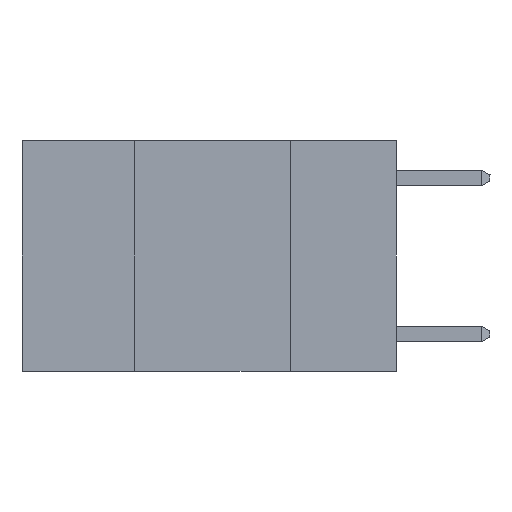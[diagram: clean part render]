
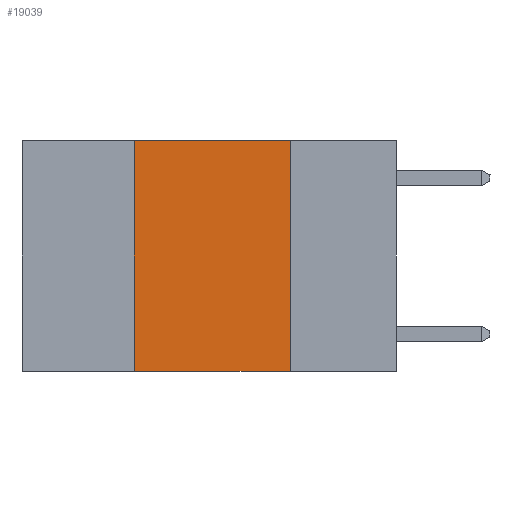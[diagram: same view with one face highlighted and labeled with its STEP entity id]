
A CAD part, left-side view. The second image highlights one B-rep face of the part: STEP entity #19039.
In plain terms, the highlighted planar face has unit normal (-1, 0, 0).
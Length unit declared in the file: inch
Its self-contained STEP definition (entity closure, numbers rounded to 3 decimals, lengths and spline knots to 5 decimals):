
#1500 = CARTESIAN_POINT ( 'NONE',  ( 0., 0.6, -0.37 ) ) ;
#1805 = EDGE_CURVE ( 'NONE', #14149, #16679, #2577, .T. ) ;
#2020 = CARTESIAN_POINT ( 'NONE',  ( 0., 0.42, -0.37 ) ) ;
#2577 = LINE ( 'NONE', #16884, #18475 ) ;
#2662 = ORIENTED_EDGE ( 'NONE', *, *, #11270, .T. ) ;
#3321 = LINE ( 'NONE', #1500, #19253 ) ;
#4371 = CARTESIAN_POINT ( 'NONE',  ( 0., 0.42, 0. ) ) ;
#4613 = DIRECTION ( 'NONE',  ( 0., -1., 0. ) ) ;
#5341 = VECTOR ( 'NONE', #7703, 39.37008 ) ;
#5435 = EDGE_CURVE ( 'NONE', #5509, #14876, #9414, .T. ) ;
#5509 = VERTEX_POINT ( 'NONE', #14030 ) ;
#7008 = EDGE_CURVE ( 'NONE', #16679, #5509, #19397, .T. ) ;
#7703 = DIRECTION ( 'NONE',  ( 0., 0., -1. ) ) ;
#9180 = CARTESIAN_POINT ( 'NONE',  ( 0., 0.17, 0. ) ) ;
#9298 = ORIENTED_EDGE ( 'NONE', *, *, #1805, .F. ) ;
#9414 = LINE ( 'NONE', #9180, #5341 ) ;
#10000 = DIRECTION ( 'NONE',  ( 0., 0., -1. ) ) ;
#10305 = FACE_OUTER_BOUND ( 'NONE', #14458, .T. ) ;
#11003 = CARTESIAN_POINT ( 'NONE',  ( 0., 0.17, -0.37 ) ) ;
#11150 = ORIENTED_EDGE ( 'NONE', *, *, #5435, .F. ) ;
#11270 = EDGE_CURVE ( 'NONE', #14149, #14876, #3321, .T. ) ;
#11470 = PLANE ( 'NONE',  #12881 ) ;
#12881 = AXIS2_PLACEMENT_3D ( 'NONE', #14586, #19259, #10000 ) ;
#14030 = CARTESIAN_POINT ( 'NONE',  ( 0., 0.17, 0. ) ) ;
#14116 = DIRECTION ( 'NONE',  ( 0., 0., 1. ) ) ;
#14149 = VERTEX_POINT ( 'NONE', #2020 ) ;
#14314 = CARTESIAN_POINT ( 'NONE',  ( 0., 0.6, 0. ) ) ;
#14458 = EDGE_LOOP ( 'NONE', ( #11150, #19744, #9298, #2662 ) ) ;
#14586 = CARTESIAN_POINT ( 'NONE',  ( 0., 0.6, 0. ) ) ;
#14876 = VERTEX_POINT ( 'NONE', #11003 ) ;
#15265 = VECTOR ( 'NONE', #18996, 39.37008 ) ;
#16679 = VERTEX_POINT ( 'NONE', #4371 ) ;
#16884 = CARTESIAN_POINT ( 'NONE',  ( 0., 0.42, 0. ) ) ;
#18475 = VECTOR ( 'NONE', #14116, 39.37008 ) ;
#18996 = DIRECTION ( 'NONE',  ( 0., -1., 0. ) ) ;
#19039 = ADVANCED_FACE ( 'NONE', ( #10305 ), #11470, .F. ) ;
#19253 = VECTOR ( 'NONE', #4613, 39.37008 ) ;
#19259 = DIRECTION ( 'NONE',  ( 1., 0., 0. ) ) ;
#19397 = LINE ( 'NONE', #14314, #15265 ) ;
#19744 = ORIENTED_EDGE ( 'NONE', *, *, #7008, .F. ) ;
